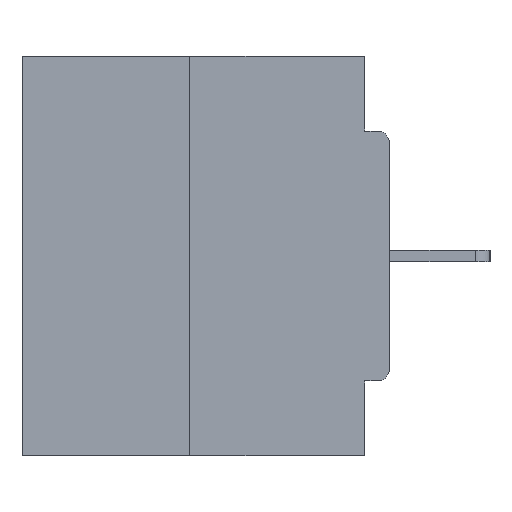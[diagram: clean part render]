
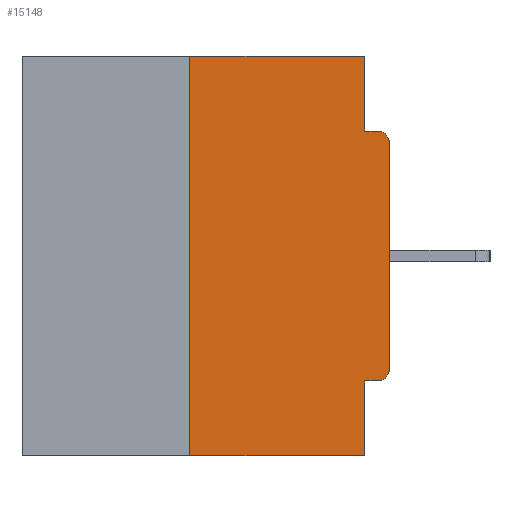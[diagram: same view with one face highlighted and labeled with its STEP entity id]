
A CAD part, left-side view. The second image highlights one B-rep face of the part: STEP entity #15148.
In plain terms, the highlighted planar face has unit normal (-1, 0, 0).
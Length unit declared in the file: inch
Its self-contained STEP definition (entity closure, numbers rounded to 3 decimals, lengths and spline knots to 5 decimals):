
#669 = LINE ( 'NONE', #10471, #9029 ) ;
#692 = VERTEX_POINT ( 'NONE', #10617 ) ;
#756 = ORIENTED_EDGE ( 'NONE', *, *, #30121, .F. ) ;
#840 = CARTESIAN_POINT ( 'NONE',  ( 0., 0., -0.0935 ) ) ;
#884 = ORIENTED_EDGE ( 'NONE', *, *, #26000, .T. ) ;
#1131 = VECTOR ( 'NONE', #9546, 39.37008 ) ;
#1290 = VECTOR ( 'NONE', #13088, 39.37008 ) ;
#2305 = ORIENTED_EDGE ( 'NONE', *, *, #18672, .F. ) ;
#2445 = ORIENTED_EDGE ( 'NONE', *, *, #17840, .F. ) ;
#2980 = VECTOR ( 'NONE', #15548, 39.37008 ) ;
#3119 = EDGE_CURVE ( 'NONE', #25532, #692, #20241, .T. ) ;
#3461 = ORIENTED_EDGE ( 'NONE', *, *, #14604, .F. ) ;
#3635 = VERTEX_POINT ( 'NONE', #24183 ) ;
#4623 = EDGE_CURVE ( 'NONE', #23724, #13651, #24522, .T. ) ;
#5514 = EDGE_LOOP ( 'NONE', ( #2305, #756, #17316, #3461, #2445, #884, #6980, #31849, #7660, #10574 ) ) ;
#5583 = VERTEX_POINT ( 'NONE', #22178 ) ;
#6652 = DIRECTION ( 'NONE',  ( -1., 0., 0. ) ) ;
#6980 = ORIENTED_EDGE ( 'NONE', *, *, #26190, .T. ) ;
#7082 = VERTEX_POINT ( 'NONE', #27975 ) ;
#7660 = ORIENTED_EDGE ( 'NONE', *, *, #22611, .F. ) ;
#7755 = DIRECTION ( 'NONE',  ( 0., 0., -1. ) ) ;
#8668 = PLANE ( 'NONE',  #20906 ) ;
#8813 = CARTESIAN_POINT ( 'NONE',  ( 0., 0.031, 0. ) ) ;
#8832 = FACE_OUTER_BOUND ( 'NONE', #5514, .T. ) ;
#9029 = VECTOR ( 'NONE', #7755, 39.37008 ) ;
#9216 = CARTESIAN_POINT ( 'NONE',  ( 0., 0.46, 0. ) ) ;
#9363 = VERTEX_POINT ( 'NONE', #24603 ) ;
#9546 = DIRECTION ( 'NONE',  ( 0., 0., 1. ) ) ;
#10471 = CARTESIAN_POINT ( 'NONE',  ( 0., 0.031, -0.5 ) ) ;
#10574 = ORIENTED_EDGE ( 'NONE', *, *, #3119, .F. ) ;
#10617 = CARTESIAN_POINT ( 'NONE',  ( 0., 0.031, -0.0935 ) ) ;
#10993 = CARTESIAN_POINT ( 'NONE',  ( 0., 0.031, 0. ) ) ;
#11619 = LINE ( 'NONE', #9216, #25135 ) ;
#12939 = EDGE_CURVE ( 'NONE', #9363, #5583, #27237, .T. ) ;
#13088 = DIRECTION ( 'NONE',  ( 0., 0., 1. ) ) ;
#13414 = DIRECTION ( 'NONE',  ( 0., 0., -1. ) ) ;
#13448 = CARTESIAN_POINT ( 'NONE',  ( 0., 0.015, -0.3915 ) ) ;
#13510 = DIRECTION ( 'NONE',  ( 1., 0., 0. ) ) ;
#13651 = VERTEX_POINT ( 'NONE', #19999 ) ;
#13681 = DIRECTION ( 'NONE',  ( 0., 0., -1. ) ) ;
#14191 = DIRECTION ( 'NONE',  ( 0., -1., 0. ) ) ;
#14495 = DIRECTION ( 'NONE',  ( 0., 1., 0. ) ) ;
#14604 = EDGE_CURVE ( 'NONE', #15623, #13651, #669, .T. ) ;
#14868 = LINE ( 'NONE', #31679, #1131 ) ;
#14960 = VECTOR ( 'NONE', #15524, 39.37008 ) ;
#15148 = ADVANCED_FACE ( 'NONE', ( #8832 ), #8668, .F. ) ;
#15359 = LINE ( 'NONE', #840, #14960 ) ;
#15524 = DIRECTION ( 'NONE',  ( 0., -1., 0. ) ) ;
#15548 = DIRECTION ( 'NONE',  ( 0., 0., -1. ) ) ;
#15623 = VERTEX_POINT ( 'NONE', #18969 ) ;
#15692 = CIRCLE ( 'NONE', #25512, 0.015 ) ;
#16343 = VECTOR ( 'NONE', #14495, 39.37008 ) ;
#16668 = DIRECTION ( 'NONE',  ( 0., -1., 0. ) ) ;
#17316 = ORIENTED_EDGE ( 'NONE', *, *, #4623, .T. ) ;
#17840 = EDGE_CURVE ( 'NONE', #3635, #15623, #29044, .T. ) ;
#18672 = EDGE_CURVE ( 'NONE', #7082, #25532, #11619, .T. ) ;
#18969 = CARTESIAN_POINT ( 'NONE',  ( 0., 0.031, -0.4065 ) ) ;
#19910 = CARTESIAN_POINT ( 'NONE',  ( 0., 0., 0. ) ) ;
#19999 = CARTESIAN_POINT ( 'NONE',  ( 0., 0.031, -0.5 ) ) ;
#20241 = LINE ( 'NONE', #10993, #2980 ) ;
#20906 = AXIS2_PLACEMENT_3D ( 'NONE', #28058, #13510, #13681 ) ;
#21387 = DIRECTION ( 'NONE',  ( -1., 0., 0. ) ) ;
#21620 = CARTESIAN_POINT ( 'NONE',  ( 0., 0.46, -0.5 ) ) ;
#22178 = CARTESIAN_POINT ( 'NONE',  ( 0., 0.015, -0.0935 ) ) ;
#22611 = EDGE_CURVE ( 'NONE', #692, #5583, #15359, .T. ) ;
#23058 = CARTESIAN_POINT ( 'NONE',  ( 0., 0., -0.3915 ) ) ;
#23724 = VERTEX_POINT ( 'NONE', #27171 ) ;
#23959 = DIRECTION ( 'NONE',  ( 0., 0., -1. ) ) ;
#24183 = CARTESIAN_POINT ( 'NONE',  ( 0., 0.015, -0.4065 ) ) ;
#24522 = LINE ( 'NONE', #21620, #29507 ) ;
#24603 = CARTESIAN_POINT ( 'NONE',  ( 0., 0., -0.1085 ) ) ;
#25135 = VECTOR ( 'NONE', #16668, 39.37008 ) ;
#25512 = AXIS2_PLACEMENT_3D ( 'NONE', #13448, #21387, #23959 ) ;
#25532 = VERTEX_POINT ( 'NONE', #8813 ) ;
#26000 = EDGE_CURVE ( 'NONE', #3635, #30816, #15692, .T. ) ;
#26190 = EDGE_CURVE ( 'NONE', #30816, #9363, #30398, .T. ) ;
#27171 = CARTESIAN_POINT ( 'NONE',  ( 0., 0.25, -0.5 ) ) ;
#27237 = CIRCLE ( 'NONE', #31884, 0.015 ) ;
#27975 = CARTESIAN_POINT ( 'NONE',  ( 0., 0.25, 0. ) ) ;
#28058 = CARTESIAN_POINT ( 'NONE',  ( 0., 0.46, 0. ) ) ;
#28762 = CARTESIAN_POINT ( 'NONE',  ( 0., 0.015, -0.1085 ) ) ;
#28872 = CARTESIAN_POINT ( 'NONE',  ( 0., 0., -0.4065 ) ) ;
#29044 = LINE ( 'NONE', #28872, #16343 ) ;
#29507 = VECTOR ( 'NONE', #14191, 39.37008 ) ;
#30121 = EDGE_CURVE ( 'NONE', #23724, #7082, #14868, .T. ) ;
#30398 = LINE ( 'NONE', #19910, #1290 ) ;
#30816 = VERTEX_POINT ( 'NONE', #23058 ) ;
#31679 = CARTESIAN_POINT ( 'NONE',  ( 0., 0.25, 0. ) ) ;
#31849 = ORIENTED_EDGE ( 'NONE', *, *, #12939, .T. ) ;
#31884 = AXIS2_PLACEMENT_3D ( 'NONE', #28762, #6652, #13414 ) ;
